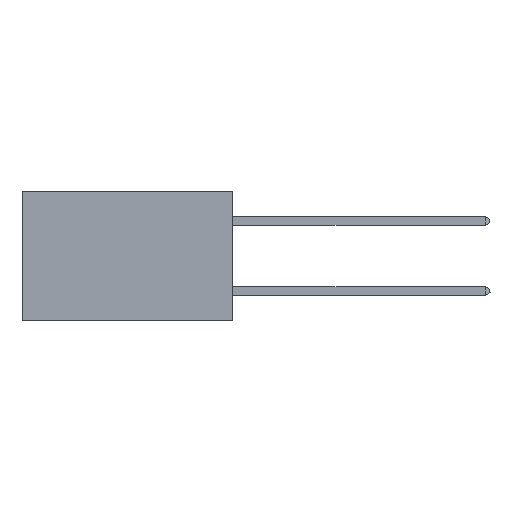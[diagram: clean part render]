
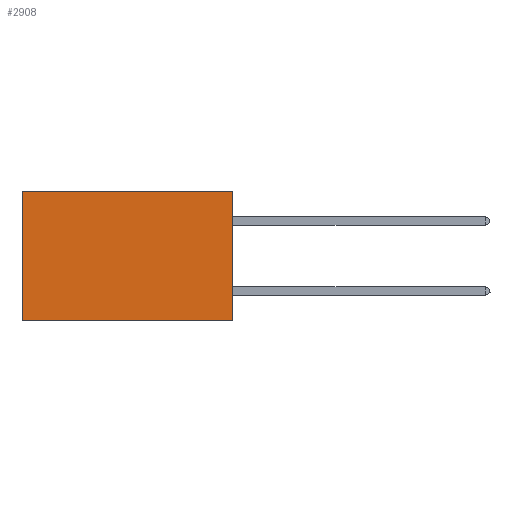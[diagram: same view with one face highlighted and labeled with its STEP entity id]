
A CAD part, left-side view. The second image highlights one B-rep face of the part: STEP entity #2908.
In plain terms, the highlighted planar face has unit normal (-1, 0, 0).
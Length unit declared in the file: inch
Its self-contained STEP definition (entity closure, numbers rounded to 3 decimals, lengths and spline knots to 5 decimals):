
#163 = CARTESIAN_POINT ( 'NONE',  ( 0.2875, 0., 0. ) ) ;
#194 = ORIENTED_EDGE ( 'NONE', *, *, #2906, .F. ) ;
#738 = EDGE_LOOP ( 'NONE', ( #3764, #194, #5441, #9330 ) ) ;
#1082 = FACE_OUTER_BOUND ( 'NONE', #738, .T. ) ;
#1428 = LINE ( 'NONE', #5819, #8869 ) ;
#1875 = PLANE ( 'NONE',  #5381 ) ;
#2103 = VERTEX_POINT ( 'NONE', #9909 ) ;
#2906 = EDGE_CURVE ( 'NONE', #3989, #3781, #10199, .T. ) ;
#2908 = ADVANCED_FACE ( 'NONE', ( #1082 ), #1875, .F. ) ;
#3184 = DIRECTION ( 'NONE',  ( 0., 0., -1. ) ) ;
#3344 = VECTOR ( 'NONE', #7016, 39.37008 ) ;
#3629 = DIRECTION ( 'NONE',  ( 0., 0., -1. ) ) ;
#3764 = ORIENTED_EDGE ( 'NONE', *, *, #4657, .T. ) ;
#3781 = VERTEX_POINT ( 'NONE', #4239 ) ;
#3864 = DIRECTION ( 'NONE',  ( 0., 1., 0. ) ) ;
#3989 = VERTEX_POINT ( 'NONE', #8354 ) ;
#4239 = CARTESIAN_POINT ( 'NONE',  ( 0.2875, 0.6, -0.37 ) ) ;
#4240 = VECTOR ( 'NONE', #3864, 39.37008 ) ;
#4403 = DIRECTION ( 'NONE',  ( 0., 0., -1. ) ) ;
#4575 = VECTOR ( 'NONE', #3629, 39.37008 ) ;
#4657 = EDGE_CURVE ( 'NONE', #2103, #3781, #1428, .T. ) ;
#5303 = DIRECTION ( 'NONE',  ( 1., 0., 0. ) ) ;
#5381 = AXIS2_PLACEMENT_3D ( 'NONE', #6069, #5303, #4403 ) ;
#5441 = ORIENTED_EDGE ( 'NONE', *, *, #8575, .F. ) ;
#5819 = CARTESIAN_POINT ( 'NONE',  ( 0.2875, 0.6, 0. ) ) ;
#6069 = CARTESIAN_POINT ( 'NONE',  ( 0.2875, 0., 0. ) ) ;
#6349 = LINE ( 'NONE', #10672, #4240 ) ;
#7016 = DIRECTION ( 'NONE',  ( 0., 1., 0. ) ) ;
#7677 = CARTESIAN_POINT ( 'NONE',  ( 0.2875, 0., -0.37 ) ) ;
#8274 = EDGE_CURVE ( 'NONE', #11047, #2103, #6349, .T. ) ;
#8354 = CARTESIAN_POINT ( 'NONE',  ( 0.2875, 0., -0.37 ) ) ;
#8575 = EDGE_CURVE ( 'NONE', #11047, #3989, #10971, .T. ) ;
#8869 = VECTOR ( 'NONE', #3184, 39.37008 ) ;
#8901 = CARTESIAN_POINT ( 'NONE',  ( 0.2875, 0., 0. ) ) ;
#9330 = ORIENTED_EDGE ( 'NONE', *, *, #8274, .T. ) ;
#9909 = CARTESIAN_POINT ( 'NONE',  ( 0.2875, 0.6, 0. ) ) ;
#10199 = LINE ( 'NONE', #7677, #3344 ) ;
#10672 = CARTESIAN_POINT ( 'NONE',  ( 0.2875, 0., 0. ) ) ;
#10971 = LINE ( 'NONE', #163, #4575 ) ;
#11047 = VERTEX_POINT ( 'NONE', #8901 ) ;
